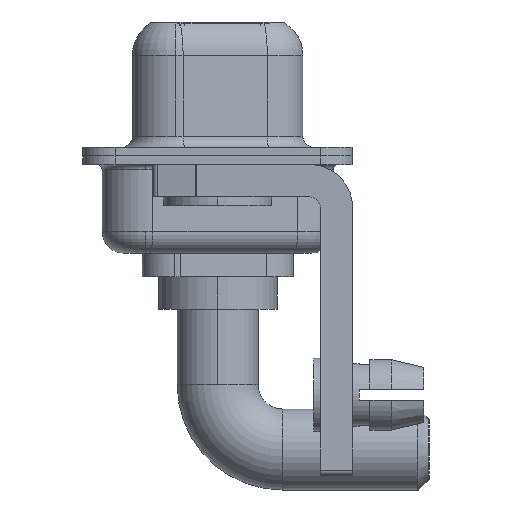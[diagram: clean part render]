
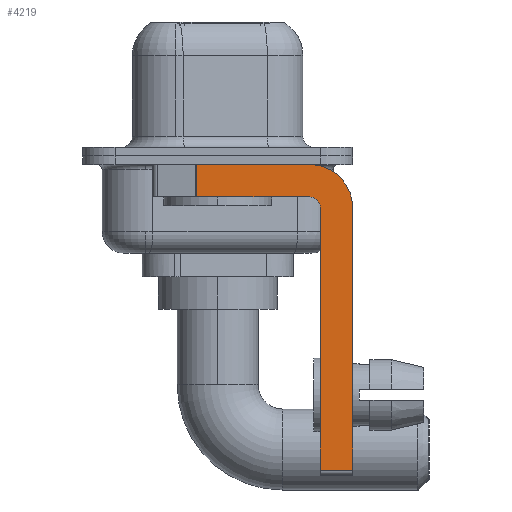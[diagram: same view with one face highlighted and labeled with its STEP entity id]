
A CAD part, left-side view. The second image highlights one B-rep face of the part: STEP entity #4219.
In plain terms, the highlighted planar face has unit normal (-1, 0, 0).
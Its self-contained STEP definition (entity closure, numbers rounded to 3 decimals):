
#321 = CARTESIAN_POINT ( 'NONE',  ( -2.9, -4.25, -2.4 ) ) ;
#562 = FACE_OUTER_BOUND ( 'NONE', #13573, .T. ) ;
#703 = CARTESIAN_POINT ( 'NONE',  ( -2.9, 0.978, -1.9 ) ) ;
#773 = ORIENTED_EDGE ( 'NONE', *, *, #5497, .F. ) ;
#919 = CARTESIAN_POINT ( 'NONE',  ( -2.9, -4.75, -14.55 ) ) ;
#1008 = LINE ( 'NONE', #4773, #6277 ) ;
#1283 = CARTESIAN_POINT ( 'NONE',  ( -2.9, 0.978, -1.9 ) ) ;
#1312 = DIRECTION ( 'NONE',  ( 0., 0., -1. ) ) ;
#1630 = VERTEX_POINT ( 'NONE', #9242 ) ;
#2249 = DIRECTION ( 'NONE',  ( 0., 0., -1. ) ) ;
#2307 = CARTESIAN_POINT ( 'NONE',  ( -2.9, -4.25, -1.9 ) ) ;
#2456 = LINE ( 'NONE', #7679, #9499 ) ;
#2951 = CIRCLE ( 'NONE', #4240, 0.5 ) ;
#2985 = CARTESIAN_POINT ( 'NONE',  ( -2.9, 0.978, -0.4 ) ) ;
#3366 = ORIENTED_EDGE ( 'NONE', *, *, #5161, .F. ) ;
#3372 = ORIENTED_EDGE ( 'NONE', *, *, #5965, .F. ) ;
#3413 = DIRECTION ( 'NONE',  ( 0., -1., 0. ) ) ;
#3543 = VERTEX_POINT ( 'NONE', #919 ) ;
#3548 = CARTESIAN_POINT ( 'NONE',  ( -2.9, -4.25, -2.4 ) ) ;
#3696 = LINE ( 'NONE', #2307, #14625 ) ;
#4213 = LINE ( 'NONE', #703, #11442 ) ;
#4219 = ADVANCED_FACE ( 'NONE', ( #562 ), #6861, .F. ) ;
#4240 = AXIS2_PLACEMENT_3D ( 'NONE', #9229, #15539, #13158 ) ;
#4249 = VERTEX_POINT ( 'NONE', #6779 ) ;
#4536 = VECTOR ( 'NONE', #3413, 1000. ) ;
#4580 = LINE ( 'NONE', #14633, #4536 ) ;
#4773 = CARTESIAN_POINT ( 'NONE',  ( -2.9, 3., -0.4 ) ) ;
#4984 = CIRCLE ( 'NONE', #10958, 2. ) ;
#5019 = CARTESIAN_POINT ( 'NONE',  ( -2.9, -4.25, -1.9 ) ) ;
#5161 = EDGE_CURVE ( 'NONE', #7561, #6074, #2951, .T. ) ;
#5497 = EDGE_CURVE ( 'NONE', #4249, #12850, #2456, .T. ) ;
#5965 = EDGE_CURVE ( 'NONE', #9484, #1630, #1008, .T. ) ;
#6074 = VERTEX_POINT ( 'NONE', #5019 ) ;
#6188 = CARTESIAN_POINT ( 'NONE',  ( -2.9, -6.25, -14.55 ) ) ;
#6277 = VECTOR ( 'NONE', #7387, 1000. ) ;
#6466 = EDGE_CURVE ( 'NONE', #9484, #12885, #4213, .T. ) ;
#6779 = CARTESIAN_POINT ( 'NONE',  ( -2.9, -6.25, -2.4 ) ) ;
#6804 = EDGE_CURVE ( 'NONE', #6074, #12885, #3696, .T. ) ;
#6861 = PLANE ( 'NONE',  #14474 ) ;
#6907 = ORIENTED_EDGE ( 'NONE', *, *, #6804, .F. ) ;
#7387 = DIRECTION ( 'NONE',  ( 0., -1., 0. ) ) ;
#7526 = CARTESIAN_POINT ( 'NONE',  ( -2.9, -4.75, -2.4 ) ) ;
#7561 = VERTEX_POINT ( 'NONE', #7526 ) ;
#7679 = CARTESIAN_POINT ( 'NONE',  ( -2.9, -6.25, -2.4 ) ) ;
#7804 = EDGE_CURVE ( 'NONE', #1630, #4249, #4984, .T. ) ;
#7832 = DIRECTION ( 'NONE',  ( 1., 0., 0. ) ) ;
#8351 = DIRECTION ( 'NONE',  ( 0., 1., 0. ) ) ;
#8782 = DIRECTION ( 'NONE',  ( 1., 0., 0. ) ) ;
#9229 = CARTESIAN_POINT ( 'NONE',  ( -2.9, -4.25, -2.4 ) ) ;
#9242 = CARTESIAN_POINT ( 'NONE',  ( -2.9, -4.25, -0.4 ) ) ;
#9424 = DIRECTION ( 'NONE',  ( 0., 0., -1. ) ) ;
#9484 = VERTEX_POINT ( 'NONE', #2985 ) ;
#9499 = VECTOR ( 'NONE', #1312, 1000. ) ;
#9649 = ORIENTED_EDGE ( 'NONE', *, *, #6466, .T. ) ;
#10483 = VECTOR ( 'NONE', #15151, 1000. ) ;
#10958 = AXIS2_PLACEMENT_3D ( 'NONE', #3548, #8782, #2249 ) ;
#11171 = ORIENTED_EDGE ( 'NONE', *, *, #11355, .F. ) ;
#11355 = EDGE_CURVE ( 'NONE', #3543, #7561, #13833, .T. ) ;
#11442 = VECTOR ( 'NONE', #9424, 1000. ) ;
#12245 = EDGE_CURVE ( 'NONE', #3543, #12850, #4580, .T. ) ;
#12754 = CARTESIAN_POINT ( 'NONE',  ( -2.9, -4.75, -14.8 ) ) ;
#12850 = VERTEX_POINT ( 'NONE', #6188 ) ;
#12885 = VERTEX_POINT ( 'NONE', #1283 ) ;
#13158 = DIRECTION ( 'NONE',  ( 0., 0., 1. ) ) ;
#13176 = ORIENTED_EDGE ( 'NONE', *, *, #7804, .F. ) ;
#13573 = EDGE_LOOP ( 'NONE', ( #3372, #9649, #6907, #3366, #11171, #14116, #773, #13176 ) ) ;
#13833 = LINE ( 'NONE', #12754, #10483 ) ;
#14116 = ORIENTED_EDGE ( 'NONE', *, *, #12245, .T. ) ;
#14474 = AXIS2_PLACEMENT_3D ( 'NONE', #321, #7832, #15270 ) ;
#14625 = VECTOR ( 'NONE', #8351, 1000. ) ;
#14633 = CARTESIAN_POINT ( 'NONE',  ( -2.9, -4.25, -14.55 ) ) ;
#15151 = DIRECTION ( 'NONE',  ( 0., 0., 1. ) ) ;
#15270 = DIRECTION ( 'NONE',  ( 0., 0., -1. ) ) ;
#15539 = DIRECTION ( 'NONE',  ( -1., 0., 0. ) ) ;
